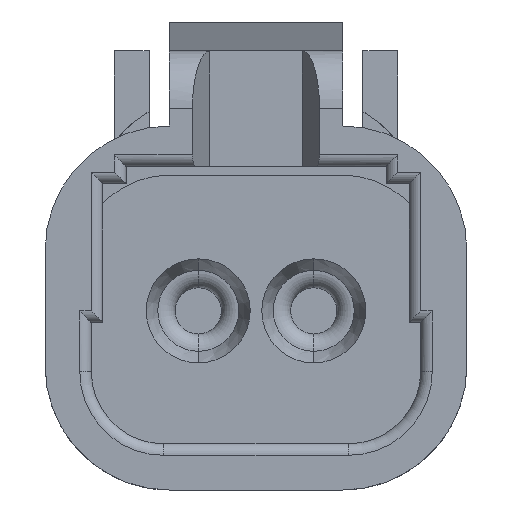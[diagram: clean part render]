
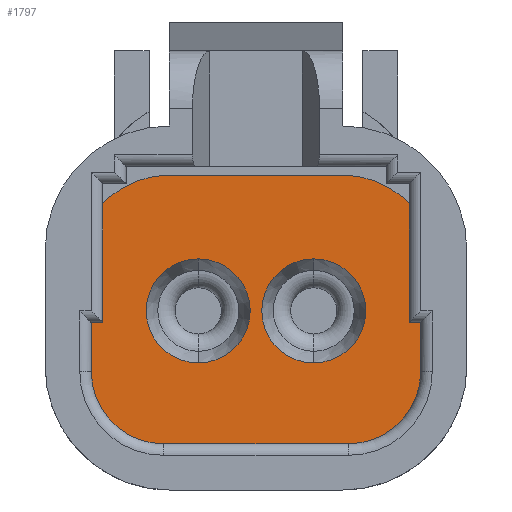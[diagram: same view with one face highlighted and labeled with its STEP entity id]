
A CAD part, front view. The second image highlights one B-rep face of the part: STEP entity #1797.
In plain terms, the highlighted planar face has unit normal (0, -1, 0).
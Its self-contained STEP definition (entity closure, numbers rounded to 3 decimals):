
#76 = EDGE_CURVE ( 'NONE', #4052, #7138, #2610, .T. ) ;
#123 = EDGE_CURVE ( 'NONE', #9188, #10654, #1046, .T. ) ;
#138 = EDGE_CURVE ( 'NONE', #4052, #8314, #7305, .T. ) ;
#317 = EDGE_CURVE ( 'NONE', #6877, #2049, #747, .T. ) ;
#498 = CARTESIAN_POINT ( 'NONE',  ( 6.579, 2.771, 9.948 ) ) ;
#555 = DIRECTION ( 'NONE',  ( 0., 0., -1. ) ) ;
#714 = DIRECTION ( 'NONE',  ( 0., 0., -1. ) ) ;
#747 = CIRCLE ( 'NONE', #10552, 1.6 ) ;
#863 = DIRECTION ( 'NONE',  ( 1., 0., 0. ) ) ;
#874 = DIRECTION ( 'NONE',  ( 0., 0., -1. ) ) ;
#1046 = CIRCLE ( 'NONE', #9784, 0.9 ) ;
#1049 = ORIENTED_EDGE ( 'NONE', *, *, #317, .T. ) ;
#1052 = CARTESIAN_POINT ( 'NONE',  ( 2.479, 2.771, 7.598 ) ) ;
#1143 = CIRCLE ( 'NONE', #9350, 0.9 ) ;
#1223 = VERTEX_POINT ( 'NONE', #4062 ) ;
#1259 = CIRCLE ( 'NONE', #7155, 0.9 ) ;
#1276 = ORIENTED_EDGE ( 'NONE', *, *, #4442, .F. ) ;
#1300 = EDGE_CURVE ( 'NONE', #4859, #2049, #6764, .T. ) ;
#1551 = CARTESIAN_POINT ( 'NONE',  ( 2.479, 2.771, 12.298 ) ) ;
#1651 = ORIENTED_EDGE ( 'NONE', *, *, #4622, .F. ) ;
#1749 = EDGE_CURVE ( 'NONE', #6877, #8314, #4104, .T. ) ;
#1759 = FACE_BOUND ( 'NONE', #9280, .T. ) ;
#1764 = DIRECTION ( 'NONE',  ( 0., 0., -1. ) ) ;
#1769 = DIRECTION ( 'NONE',  ( 0., 0., 1. ) ) ;
#1797 = ADVANCED_FACE ( 'NONE', ( #1759, #6284, #4371 ), #7793, .F. ) ;
#2030 = DIRECTION ( 'NONE',  ( 0., 0., 1. ) ) ;
#2049 = VERTEX_POINT ( 'NONE', #5616 ) ;
#2292 = EDGE_LOOP ( 'NONE', ( #9027, #1276 ) ) ;
#2328 = CIRCLE ( 'NONE', #3572, 1.6 ) ;
#2362 = CARTESIAN_POINT ( 'NONE',  ( 4.079, 2.771, 12.298 ) ) ;
#2476 = AXIS2_PLACEMENT_3D ( 'NONE', #3293, #9425, #1769 ) ;
#2610 = LINE ( 'NONE', #7547, #10681 ) ;
#2836 = DIRECTION ( 'NONE',  ( 0., -1., 0. ) ) ;
#2892 = DIRECTION ( 'NONE',  ( 0., 0., 1. ) ) ;
#3004 = DIRECTION ( 'NONE',  ( 0., -1., 0. ) ) ;
#3054 = CARTESIAN_POINT ( 'NONE',  ( 7.079, 2.771, 7.598 ) ) ;
#3293 = CARTESIAN_POINT ( 'NONE',  ( 7.079, 2.771, 10.698 ) ) ;
#3401 = CARTESIAN_POINT ( 'NONE',  ( 2.479, 2.771, 7.598 ) ) ;
#3499 = VECTOR ( 'NONE', #6031, 1000. ) ;
#3549 = CARTESIAN_POINT ( 'NONE',  ( 6.579, 2.771, 9.948 ) ) ;
#3572 = AXIS2_PLACEMENT_3D ( 'NONE', #10716, #2836, #2892 ) ;
#3615 = EDGE_CURVE ( 'NONE', #4859, #1223, #2328, .T. ) ;
#3725 = ORIENTED_EDGE ( 'NONE', *, *, #123, .F. ) ;
#4041 = CARTESIAN_POINT ( 'NONE',  ( 8.679, 2.771, 10.698 ) ) ;
#4052 = VERTEX_POINT ( 'NONE', #4041 ) ;
#4062 = CARTESIAN_POINT ( 'NONE',  ( 4.079, 2.771, 7.598 ) ) ;
#4100 = EDGE_LOOP ( 'NONE', ( #7992, #9664, #8621, #1049, #6650, #5625, #1651, #8726 ) ) ;
#4104 = LINE ( 'NONE', #1551, #10418 ) ;
#4121 = VERTEX_POINT ( 'NONE', #3054 ) ;
#4371 = FACE_OUTER_BOUND ( 'NONE', #4100, .T. ) ;
#4442 = EDGE_CURVE ( 'NONE', #10968, #7846, #1259, .T. ) ;
#4513 = CARTESIAN_POINT ( 'NONE',  ( 4.579, 2.771, 9.948 ) ) ;
#4622 = EDGE_CURVE ( 'NONE', #4121, #1223, #8702, .T. ) ;
#4679 = CARTESIAN_POINT ( 'NONE',  ( 7.079, 2.771, 12.298 ) ) ;
#4775 = CARTESIAN_POINT ( 'NONE',  ( 4.079, 2.771, 10.698 ) ) ;
#4859 = VERTEX_POINT ( 'NONE', #4948 ) ;
#4948 = CARTESIAN_POINT ( 'NONE',  ( 2.479, 2.771, 9.198 ) ) ;
#5375 = CARTESIAN_POINT ( 'NONE',  ( 6.579, 2.771, 9.048 ) ) ;
#5509 = DIRECTION ( 'NONE',  ( 0., 0., 1. ) ) ;
#5590 = CIRCLE ( 'NONE', #10218, 1.6 ) ;
#5616 = CARTESIAN_POINT ( 'NONE',  ( 2.479, 2.771, 10.698 ) ) ;
#5625 = ORIENTED_EDGE ( 'NONE', *, *, #3615, .T. ) ;
#5639 = CARTESIAN_POINT ( 'NONE',  ( 8.679, 2.771, 9.198 ) ) ;
#5822 = CARTESIAN_POINT ( 'NONE',  ( 6.579, 2.771, 10.848 ) ) ;
#5981 = EDGE_CURVE ( 'NONE', #10654, #9188, #10844, .T. ) ;
#6021 = DIRECTION ( 'NONE',  ( 0., -1., 0. ) ) ;
#6031 = DIRECTION ( 'NONE',  ( -1., 0., 0. ) ) ;
#6159 = CARTESIAN_POINT ( 'NONE',  ( 4.579, 2.771, 9.048 ) ) ;
#6259 = EDGE_CURVE ( 'NONE', #4121, #7138, #5590, .T. ) ;
#6284 = FACE_BOUND ( 'NONE', #2292, .T. ) ;
#6527 = DIRECTION ( 'NONE',  ( 0., 0., 1. ) ) ;
#6650 = ORIENTED_EDGE ( 'NONE', *, *, #1300, .F. ) ;
#6764 = LINE ( 'NONE', #3401, #8588 ) ;
#6871 = CARTESIAN_POINT ( 'NONE',  ( 4.579, 2.771, 9.948 ) ) ;
#6877 = VERTEX_POINT ( 'NONE', #2362 ) ;
#6927 = DIRECTION ( 'NONE',  ( 0., 0., 1. ) ) ;
#7138 = VERTEX_POINT ( 'NONE', #5639 ) ;
#7155 = AXIS2_PLACEMENT_3D ( 'NONE', #498, #10729, #555 ) ;
#7289 = EDGE_CURVE ( 'NONE', #7846, #10968, #1143, .T. ) ;
#7305 = CIRCLE ( 'NONE', #2476, 1.6 ) ;
#7469 = AXIS2_PLACEMENT_3D ( 'NONE', #4513, #7935, #9725 ) ;
#7524 = ORIENTED_EDGE ( 'NONE', *, *, #5981, .F. ) ;
#7547 = CARTESIAN_POINT ( 'NONE',  ( 8.679, 2.771, 7.598 ) ) ;
#7793 = PLANE ( 'NONE',  #9174 ) ;
#7846 = VERTEX_POINT ( 'NONE', #5375 ) ;
#7935 = DIRECTION ( 'NONE',  ( 0., -1., 0. ) ) ;
#7965 = CARTESIAN_POINT ( 'NONE',  ( 7.079, 2.771, 9.198 ) ) ;
#7992 = ORIENTED_EDGE ( 'NONE', *, *, #76, .F. ) ;
#8314 = VERTEX_POINT ( 'NONE', #4679 ) ;
#8588 = VECTOR ( 'NONE', #6927, 1000. ) ;
#8621 = ORIENTED_EDGE ( 'NONE', *, *, #1749, .F. ) ;
#8702 = LINE ( 'NONE', #1052, #3499 ) ;
#8726 = ORIENTED_EDGE ( 'NONE', *, *, #6259, .T. ) ;
#8840 = DIRECTION ( 'NONE',  ( 0., 1., 0. ) ) ;
#9027 = ORIENTED_EDGE ( 'NONE', *, *, #7289, .F. ) ;
#9174 = AXIS2_PLACEMENT_3D ( 'NONE', #10304, #8840, #2030 ) ;
#9183 = CARTESIAN_POINT ( 'NONE',  ( 4.579, 2.771, 10.848 ) ) ;
#9188 = VERTEX_POINT ( 'NONE', #9183 ) ;
#9280 = EDGE_LOOP ( 'NONE', ( #7524, #3725 ) ) ;
#9350 = AXIS2_PLACEMENT_3D ( 'NONE', #3549, #9420, #1764 ) ;
#9420 = DIRECTION ( 'NONE',  ( 0., -1., 0. ) ) ;
#9425 = DIRECTION ( 'NONE',  ( 0., -1., 0. ) ) ;
#9664 = ORIENTED_EDGE ( 'NONE', *, *, #138, .T. ) ;
#9725 = DIRECTION ( 'NONE',  ( 0., 0., -1. ) ) ;
#9784 = AXIS2_PLACEMENT_3D ( 'NONE', #6871, #6021, #714 ) ;
#10218 = AXIS2_PLACEMENT_3D ( 'NONE', #7965, #3004, #5509 ) ;
#10304 = CARTESIAN_POINT ( 'NONE',  ( 2.479, 2.771, 7.598 ) ) ;
#10418 = VECTOR ( 'NONE', #863, 1000. ) ;
#10552 = AXIS2_PLACEMENT_3D ( 'NONE', #4775, #10650, #6527 ) ;
#10650 = DIRECTION ( 'NONE',  ( 0., -1., 0. ) ) ;
#10654 = VERTEX_POINT ( 'NONE', #6159 ) ;
#10681 = VECTOR ( 'NONE', #874, 1000. ) ;
#10716 = CARTESIAN_POINT ( 'NONE',  ( 4.079, 2.771, 9.198 ) ) ;
#10729 = DIRECTION ( 'NONE',  ( 0., -1., 0. ) ) ;
#10844 = CIRCLE ( 'NONE', #7469, 0.9 ) ;
#10968 = VERTEX_POINT ( 'NONE', #5822 ) ;
